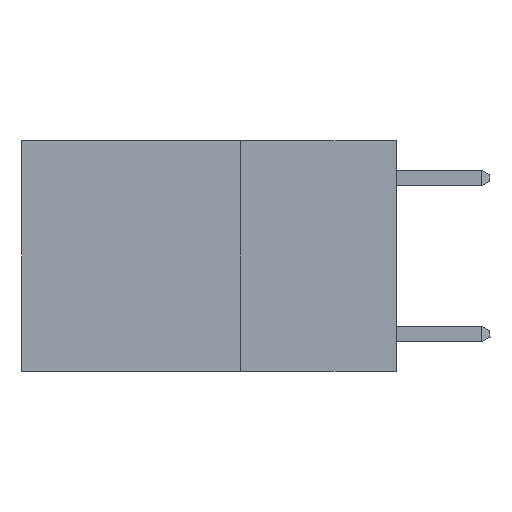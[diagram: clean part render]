
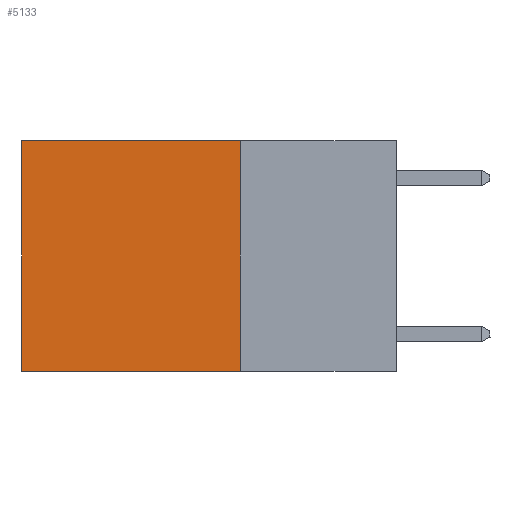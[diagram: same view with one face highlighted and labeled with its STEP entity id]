
A CAD part, left-side view. The second image highlights one B-rep face of the part: STEP entity #5133.
In plain terms, the highlighted planar face has unit normal (-1, 0, 0).
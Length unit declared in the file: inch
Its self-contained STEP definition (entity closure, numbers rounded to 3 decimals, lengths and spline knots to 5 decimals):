
#100 = CARTESIAN_POINT ( 'NONE',  ( 0.2625, 0.25, 0. ) ) ;
#877 = DIRECTION ( 'NONE',  ( 0., 1., 0. ) ) ;
#1198 = FACE_OUTER_BOUND ( 'NONE', #2621, .T. ) ;
#1564 = VERTEX_POINT ( 'NONE', #17465 ) ;
#1727 = DIRECTION ( 'NONE',  ( 0., 0., -1. ) ) ;
#2379 = LINE ( 'NONE', #7148, #12563 ) ;
#2621 = EDGE_LOOP ( 'NONE', ( #15832, #22093, #4304, #6890 ) ) ;
#4304 = ORIENTED_EDGE ( 'NONE', *, *, #9984, .F. ) ;
#4305 = EDGE_CURVE ( 'NONE', #6693, #15064, #20951, .T. ) ;
#4745 = VECTOR ( 'NONE', #16547, 39.37008 ) ;
#5133 = ADVANCED_FACE ( 'NONE', ( #1198 ), #23875, .F. ) ;
#6357 = CARTESIAN_POINT ( 'NONE',  ( 0.2625, 0.25, 0. ) ) ;
#6693 = VERTEX_POINT ( 'NONE', #18302 ) ;
#6771 = EDGE_CURVE ( 'NONE', #1564, #13112, #25907, .T. ) ;
#6890 = ORIENTED_EDGE ( 'NONE', *, *, #6771, .T. ) ;
#7148 = CARTESIAN_POINT ( 'NONE',  ( 0.2625, 0.6, 0. ) ) ;
#8084 = VECTOR ( 'NONE', #22526, 39.37008 ) ;
#8299 = EDGE_CURVE ( 'NONE', #13112, #15064, #2379, .T. ) ;
#8739 = LINE ( 'NONE', #6357, #8084 ) ;
#9984 = EDGE_CURVE ( 'NONE', #1564, #6693, #8739, .T. ) ;
#10207 = VECTOR ( 'NONE', #877, 39.37008 ) ;
#12563 = VECTOR ( 'NONE', #13288, 39.37008 ) ;
#13112 = VERTEX_POINT ( 'NONE', #15239 ) ;
#13288 = DIRECTION ( 'NONE',  ( 0., 0., -1. ) ) ;
#13930 = DIRECTION ( 'NONE',  ( 1., 0., 0. ) ) ;
#14152 = AXIS2_PLACEMENT_3D ( 'NONE', #15914, #13930, #1727 ) ;
#15064 = VERTEX_POINT ( 'NONE', #21973 ) ;
#15239 = CARTESIAN_POINT ( 'NONE',  ( 0.2625, 0.6, 0. ) ) ;
#15832 = ORIENTED_EDGE ( 'NONE', *, *, #8299, .T. ) ;
#15914 = CARTESIAN_POINT ( 'NONE',  ( 0.2625, 0.25, 0. ) ) ;
#16547 = DIRECTION ( 'NONE',  ( 0., 1., 0. ) ) ;
#17465 = CARTESIAN_POINT ( 'NONE',  ( 0.2625, 0.25, 0. ) ) ;
#18302 = CARTESIAN_POINT ( 'NONE',  ( 0.2625, 0.25, -0.37 ) ) ;
#19160 = CARTESIAN_POINT ( 'NONE',  ( 0.2625, 0.25, -0.37 ) ) ;
#20951 = LINE ( 'NONE', #19160, #10207 ) ;
#21973 = CARTESIAN_POINT ( 'NONE',  ( 0.2625, 0.6, -0.37 ) ) ;
#22093 = ORIENTED_EDGE ( 'NONE', *, *, #4305, .F. ) ;
#22526 = DIRECTION ( 'NONE',  ( 0., 0., -1. ) ) ;
#23875 = PLANE ( 'NONE',  #14152 ) ;
#25907 = LINE ( 'NONE', #100, #4745 ) ;
